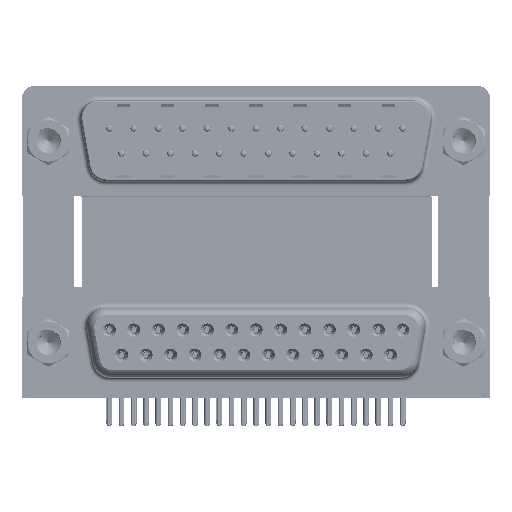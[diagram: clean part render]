
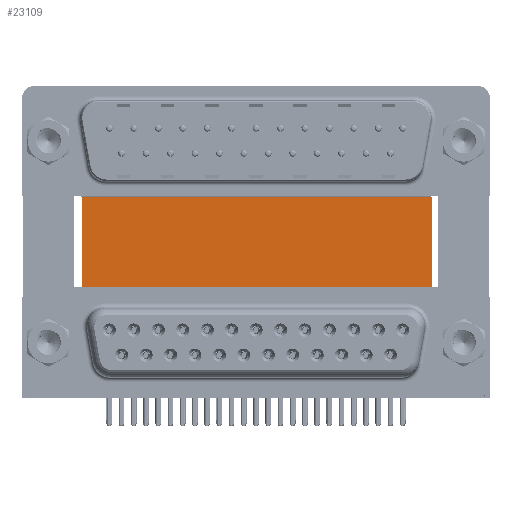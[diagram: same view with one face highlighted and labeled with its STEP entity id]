
A CAD part, top view. The second image highlights one B-rep face of the part: STEP entity #23109.
In plain terms, the highlighted planar face has unit normal (0, 0, 1).
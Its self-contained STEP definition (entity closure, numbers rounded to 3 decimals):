
#1037 = VERTEX_POINT ( 'NONE', #5412 ) ;
#1066 = ORIENTED_EDGE ( 'NONE', *, *, #54823, .T. ) ;
#3977 = CARTESIAN_POINT ( 'NONE',  ( 43.43, 16.585, -12. ) ) ;
#5412 = CARTESIAN_POINT ( 'NONE',  ( 3.79, 16.585, -12. ) ) ;
#5679 = DIRECTION ( 'NONE',  ( 0., -1., 0. ) ) ;
#5952 = CARTESIAN_POINT ( 'NONE',  ( 3.79, -3.735, -12. ) ) ;
#7871 = LINE ( 'NONE', #46873, #20801 ) ;
#10709 = LINE ( 'NONE', #57600, #58630 ) ;
#12487 = AXIS2_PLACEMENT_3D ( 'NONE', #30043, #44514, #53639 ) ;
#12836 = VERTEX_POINT ( 'NONE', #3977 ) ;
#16677 = DIRECTION ( 'NONE',  ( 0., -1., 0. ) ) ;
#17228 = DIRECTION ( 'NONE',  ( 1., 0., 0. ) ) ;
#20185 = EDGE_CURVE ( 'NONE', #12836, #56075, #60393, .T. ) ;
#20692 = EDGE_CURVE ( 'NONE', #32074, #56075, #36104, .T. ) ;
#20801 = VECTOR ( 'NONE', #56923, 1000. ) ;
#23109 = ADVANCED_FACE ( 'NONE', ( #25322 ), #28825, .F. ) ;
#24972 = EDGE_CURVE ( 'NONE', #1037, #12836, #7871, .T. ) ;
#25322 = FACE_OUTER_BOUND ( 'NONE', #55615, .T. ) ;
#28825 = PLANE ( 'NONE',  #12487 ) ;
#30043 = CARTESIAN_POINT ( 'NONE',  ( 3.79, 16.585, -12. ) ) ;
#32074 = VERTEX_POINT ( 'NONE', #5952 ) ;
#36104 = LINE ( 'NONE', #45859, #56680 ) ;
#36420 = ORIENTED_EDGE ( 'NONE', *, *, #24972, .F. ) ;
#36510 = VECTOR ( 'NONE', #16677, 1000. ) ;
#37110 = ORIENTED_EDGE ( 'NONE', *, *, #20185, .F. ) ;
#38356 = ORIENTED_EDGE ( 'NONE', *, *, #20692, .T. ) ;
#44514 = DIRECTION ( 'NONE',  ( 0., 0., -1. ) ) ;
#45859 = CARTESIAN_POINT ( 'NONE',  ( 3.79, -3.735, -12. ) ) ;
#46873 = CARTESIAN_POINT ( 'NONE',  ( 3.79, 16.585, -12. ) ) ;
#53639 = DIRECTION ( 'NONE',  ( -1., 0., 0. ) ) ;
#53924 = CARTESIAN_POINT ( 'NONE',  ( 43.43, -3.735, -12. ) ) ;
#54823 = EDGE_CURVE ( 'NONE', #1037, #32074, #10709, .T. ) ;
#55360 = CARTESIAN_POINT ( 'NONE',  ( 43.43, 16.585, -12. ) ) ;
#55615 = EDGE_LOOP ( 'NONE', ( #38356, #37110, #36420, #1066 ) ) ;
#56075 = VERTEX_POINT ( 'NONE', #53924 ) ;
#56680 = VECTOR ( 'NONE', #17228, 1000. ) ;
#56923 = DIRECTION ( 'NONE',  ( 1., 0., 0. ) ) ;
#57600 = CARTESIAN_POINT ( 'NONE',  ( 3.79, 16.585, -12. ) ) ;
#58630 = VECTOR ( 'NONE', #5679, 1000. ) ;
#60393 = LINE ( 'NONE', #55360, #36510 ) ;
